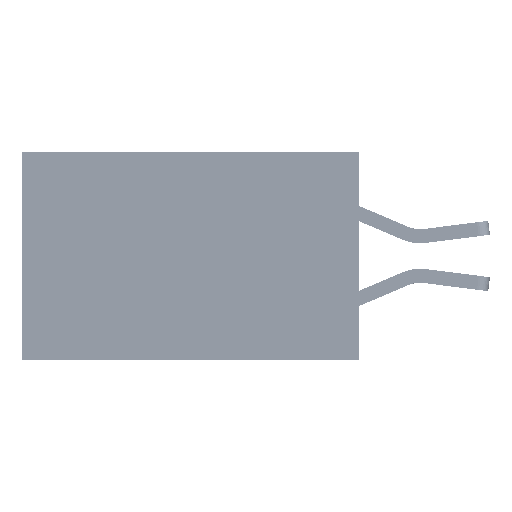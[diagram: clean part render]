
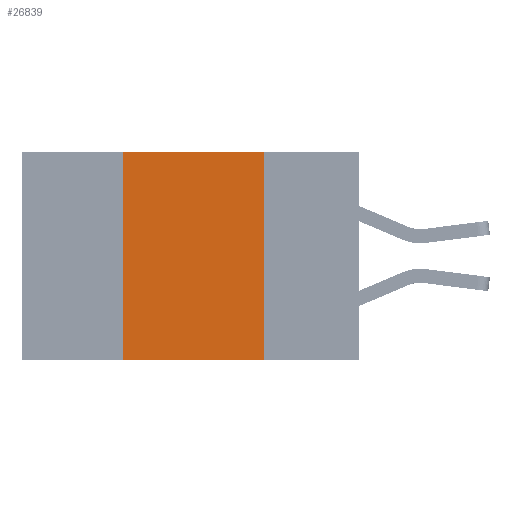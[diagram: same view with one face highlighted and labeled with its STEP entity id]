
A CAD part, left-side view. The second image highlights one B-rep face of the part: STEP entity #26839.
In plain terms, the highlighted planar face has unit normal (-1, 0, 0).
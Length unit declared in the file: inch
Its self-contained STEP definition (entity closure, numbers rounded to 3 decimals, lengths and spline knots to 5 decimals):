
#4275 = DIRECTION ( 'NONE',  ( 0., -1., 0. ) ) ;
#5500 = LINE ( 'NONE', #34398, #9677 ) ;
#6126 = ORIENTED_EDGE ( 'NONE', *, *, #44836, .F. ) ;
#9677 = VECTOR ( 'NONE', #21532, 39.37008 ) ;
#9849 = CARTESIAN_POINT ( 'NONE',  ( 0., 0.17, -0.37 ) ) ;
#9873 = ORIENTED_EDGE ( 'NONE', *, *, #20669, .F. ) ;
#11068 = ORIENTED_EDGE ( 'NONE', *, *, #45935, .T. ) ;
#11865 = CARTESIAN_POINT ( 'NONE',  ( 0., 0.42, -0.37 ) ) ;
#12534 = FACE_OUTER_BOUND ( 'NONE', #22246, .T. ) ;
#12735 = VERTEX_POINT ( 'NONE', #11865 ) ;
#12869 = EDGE_CURVE ( 'NONE', #12735, #28286, #5500, .T. ) ;
#14337 = CARTESIAN_POINT ( 'NONE',  ( 0., 0.42, 0. ) ) ;
#14503 = LINE ( 'NONE', #43459, #14808 ) ;
#14808 = VECTOR ( 'NONE', #35265, 39.37008 ) ;
#15558 = CARTESIAN_POINT ( 'NONE',  ( 0., 0.17, 0. ) ) ;
#15780 = CARTESIAN_POINT ( 'NONE',  ( 0., 0.6, -0.37 ) ) ;
#16716 = DIRECTION ( 'NONE',  ( 1., 0., 0. ) ) ;
#20669 = EDGE_CURVE ( 'NONE', #28286, #39289, #48281, .T. ) ;
#21532 = DIRECTION ( 'NONE',  ( 0., 0., 1. ) ) ;
#22246 = EDGE_LOOP ( 'NONE', ( #6126, #9873, #50045, #11068 ) ) ;
#23749 = CARTESIAN_POINT ( 'NONE',  ( 0., 0.6, 0. ) ) ;
#24418 = DIRECTION ( 'NONE',  ( 0., -1., 0. ) ) ;
#26839 = ADVANCED_FACE ( 'NONE', ( #12534 ), #28532, .F. ) ;
#27892 = AXIS2_PLACEMENT_3D ( 'NONE', #36706, #16716, #32747 ) ;
#28286 = VERTEX_POINT ( 'NONE', #14337 ) ;
#28532 = PLANE ( 'NONE',  #27892 ) ;
#30827 = VECTOR ( 'NONE', #24418, 39.37008 ) ;
#32747 = DIRECTION ( 'NONE',  ( 0., 0., -1. ) ) ;
#34398 = CARTESIAN_POINT ( 'NONE',  ( 0., 0.42, 0. ) ) ;
#35265 = DIRECTION ( 'NONE',  ( 0., 0., -1. ) ) ;
#36706 = CARTESIAN_POINT ( 'NONE',  ( 0., 0.6, 0. ) ) ;
#39289 = VERTEX_POINT ( 'NONE', #15558 ) ;
#42653 = VECTOR ( 'NONE', #4275, 39.37008 ) ;
#42961 = VERTEX_POINT ( 'NONE', #9849 ) ;
#43459 = CARTESIAN_POINT ( 'NONE',  ( 0., 0.17, 0. ) ) ;
#44836 = EDGE_CURVE ( 'NONE', #39289, #42961, #14503, .T. ) ;
#45935 = EDGE_CURVE ( 'NONE', #12735, #42961, #51896, .T. ) ;
#48281 = LINE ( 'NONE', #23749, #42653 ) ;
#50045 = ORIENTED_EDGE ( 'NONE', *, *, #12869, .F. ) ;
#51896 = LINE ( 'NONE', #15780, #30827 ) ;
